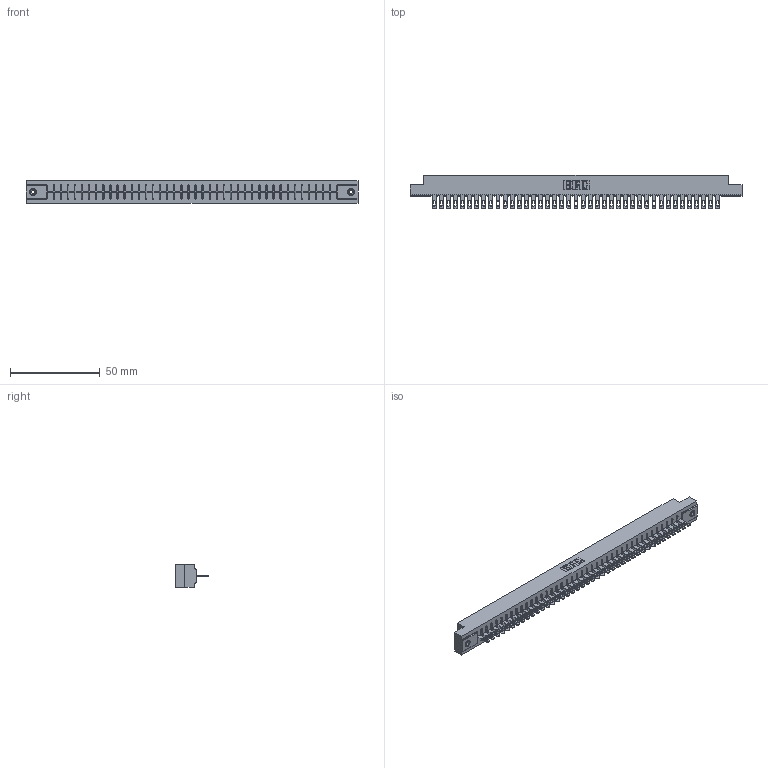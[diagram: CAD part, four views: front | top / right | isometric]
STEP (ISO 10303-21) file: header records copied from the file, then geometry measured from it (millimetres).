
FILE_DESCRIPTION (( 'STEP AP203' ), '1' );
FILE_NAME ('306-041-400-108.STEP', '2020-09-22T12:28:18', ( '' ), ( '' ), 'SwSTEP 2.0', 'SolidWorks 2020', '' );
FILE_SCHEMA (( 'CONFIG_CONTROL_DESIGN' ));
Length unit declared in the file: inch
Products named in the file (4): 306 Part_.156 Dia; 306-041-400-108; 345-250-001_345-250-003-102; 306-290-001_100
Assembly tree (44 placements, depth 2):
  306-041-400-108
    306 Part_.156 Dia
    306-290-001_100  x41
    345-250-001_345-250-003-102  x2
Bounding box: 185.47 x 18.87 x 12.7 mm (x, y, z)
Volume: 20627.3 mm3; surface area: 21909.1 mm2
Topology: 44 solids, 44 shells, 3292 faces, 9267 edges, 5950 vertices
Faces by surface type: plane 2150, cylinder 962, sphere 164, cone 12, torus 4
Entity records: 39713 total; most frequent: CARTESIAN_POINT 6649, ORIENTED_EDGE 6586, DIRECTION 6565, EDGE_CURVE 3293, LINE 2573, VECTOR 2573, VERTEX_POINT 2080, AXIS2_PLACEMENT_3D 1996
